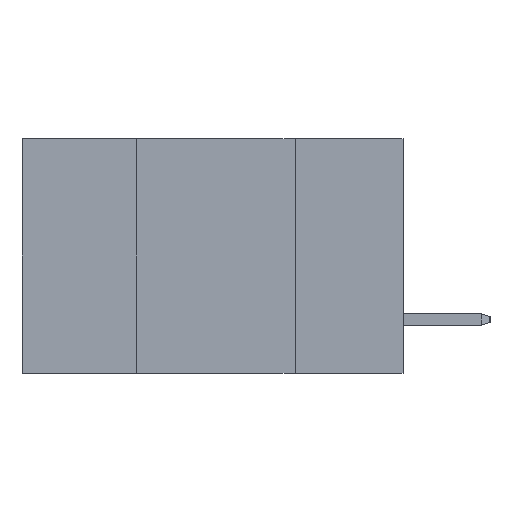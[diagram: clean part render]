
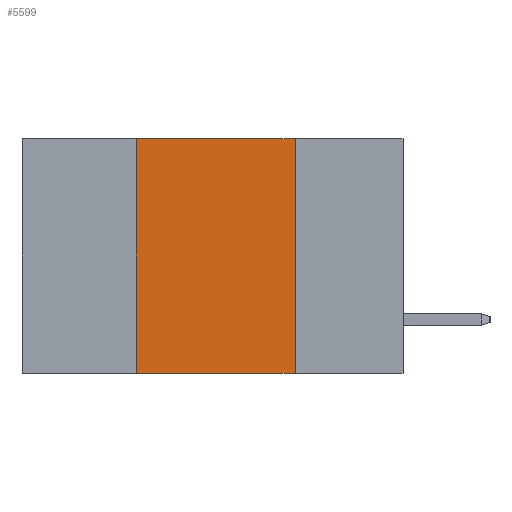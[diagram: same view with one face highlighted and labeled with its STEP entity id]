
A CAD part, left-side view. The second image highlights one B-rep face of the part: STEP entity #5599.
In plain terms, the highlighted planar face has unit normal (-1, 0, 0).
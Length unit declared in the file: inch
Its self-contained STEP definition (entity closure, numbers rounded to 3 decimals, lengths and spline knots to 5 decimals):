
#230 = CARTESIAN_POINT ( 'NONE',  ( 0., 0.17, -0.37 ) ) ;
#504 = ORIENTED_EDGE ( 'NONE', *, *, #3517, .F. ) ;
#1333 = ORIENTED_EDGE ( 'NONE', *, *, #3431, .T. ) ;
#1408 = PLANE ( 'NONE',  #3679 ) ;
#1481 = CARTESIAN_POINT ( 'NONE',  ( 0., 0.6, 0. ) ) ;
#1580 = LINE ( 'NONE', #11037, #9284 ) ;
#1713 = LINE ( 'NONE', #1785, #2360 ) ;
#1785 = CARTESIAN_POINT ( 'NONE',  ( 0., 0.42, 0. ) ) ;
#2360 = VECTOR ( 'NONE', #6022, 39.37008 ) ;
#2417 = VECTOR ( 'NONE', #6855, 39.37008 ) ;
#2531 = FACE_OUTER_BOUND ( 'NONE', #8674, .T. ) ;
#2561 = CARTESIAN_POINT ( 'NONE',  ( 0., 0.17, 0. ) ) ;
#2709 = CARTESIAN_POINT ( 'NONE',  ( 0., 0.17, 0. ) ) ;
#3261 = ORIENTED_EDGE ( 'NONE', *, *, #12979, .F. ) ;
#3431 = EDGE_CURVE ( 'NONE', #13423, #5815, #6466, .T. ) ;
#3517 = EDGE_CURVE ( 'NONE', #13593, #9814, #1580, .T. ) ;
#3679 = AXIS2_PLACEMENT_3D ( 'NONE', #1481, #11010, #6829 ) ;
#4185 = ORIENTED_EDGE ( 'NONE', *, *, #10617, .F. ) ;
#5019 = VECTOR ( 'NONE', #5414, 39.37008 ) ;
#5414 = DIRECTION ( 'NONE',  ( 0., -1., 0. ) ) ;
#5599 = ADVANCED_FACE ( 'NONE', ( #2531 ), #1408, .F. ) ;
#5815 = VERTEX_POINT ( 'NONE', #230 ) ;
#5887 = DIRECTION ( 'NONE',  ( 0., -1., 0. ) ) ;
#6022 = DIRECTION ( 'NONE',  ( 0., 0., 1. ) ) ;
#6466 = LINE ( 'NONE', #10775, #5019 ) ;
#6829 = DIRECTION ( 'NONE',  ( 0., 0., -1. ) ) ;
#6855 = DIRECTION ( 'NONE',  ( 0., 0., -1. ) ) ;
#6976 = CARTESIAN_POINT ( 'NONE',  ( 0., 0.42, -0.37 ) ) ;
#7107 = CARTESIAN_POINT ( 'NONE',  ( 0., 0.42, 0. ) ) ;
#8674 = EDGE_LOOP ( 'NONE', ( #3261, #504, #4185, #1333 ) ) ;
#9284 = VECTOR ( 'NONE', #5887, 39.37008 ) ;
#9814 = VERTEX_POINT ( 'NONE', #2709 ) ;
#10617 = EDGE_CURVE ( 'NONE', #13423, #13593, #1713, .T. ) ;
#10775 = CARTESIAN_POINT ( 'NONE',  ( 0., 0.6, -0.37 ) ) ;
#11010 = DIRECTION ( 'NONE',  ( 1., 0., 0. ) ) ;
#11037 = CARTESIAN_POINT ( 'NONE',  ( 0., 0.6, 0. ) ) ;
#12979 = EDGE_CURVE ( 'NONE', #9814, #5815, #13344, .T. ) ;
#13344 = LINE ( 'NONE', #2561, #2417 ) ;
#13423 = VERTEX_POINT ( 'NONE', #6976 ) ;
#13593 = VERTEX_POINT ( 'NONE', #7107 ) ;
